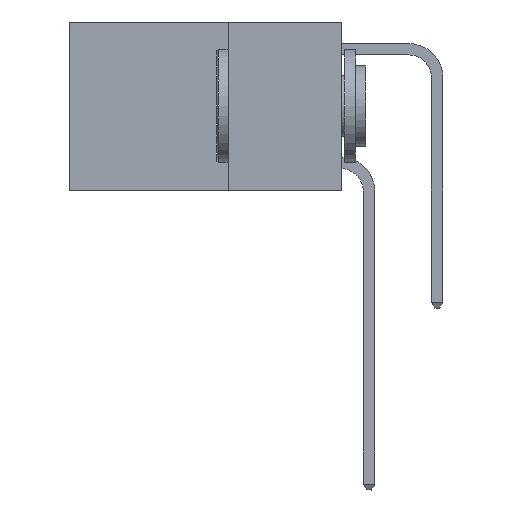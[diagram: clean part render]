
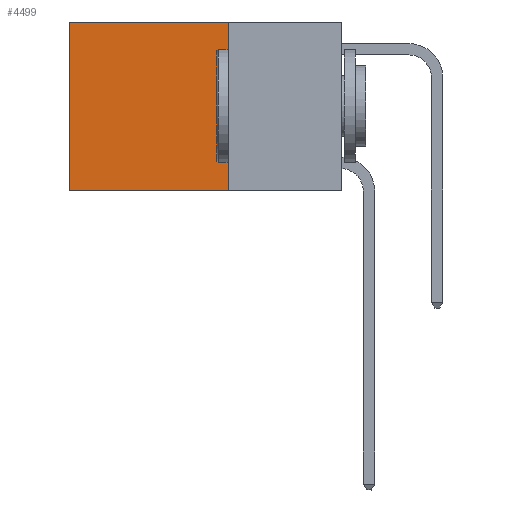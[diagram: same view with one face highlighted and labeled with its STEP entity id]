
A CAD part, left-side view. The second image highlights one B-rep face of the part: STEP entity #4499.
In plain terms, the highlighted planar face has unit normal (-1, 0, 0).
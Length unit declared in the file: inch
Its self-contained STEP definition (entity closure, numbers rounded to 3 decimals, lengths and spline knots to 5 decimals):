
#1267 = CARTESIAN_POINT ( 'NONE',  ( 0.2625, 0.25, -0.37 ) ) ;
#3978 = VECTOR ( 'NONE', #19620, 39.37008 ) ;
#4499 = ADVANCED_FACE ( 'NONE', ( #9199 ), #13347, .F. ) ;
#5817 = ORIENTED_EDGE ( 'NONE', *, *, #18738, .F. ) ;
#6195 = CARTESIAN_POINT ( 'NONE',  ( 0.2625, 0.25, 0. ) ) ;
#7428 = LINE ( 'NONE', #13682, #24692 ) ;
#7809 = CARTESIAN_POINT ( 'NONE',  ( 0.2625, 0.6, 0. ) ) ;
#7975 = LINE ( 'NONE', #7809, #18261 ) ;
#8742 = VERTEX_POINT ( 'NONE', #15320 ) ;
#9199 = FACE_OUTER_BOUND ( 'NONE', #31244, .T. ) ;
#9621 = CARTESIAN_POINT ( 'NONE',  ( 0.2625, 0.25, -0.37 ) ) ;
#10654 = EDGE_CURVE ( 'NONE', #8742, #15787, #7975, .T. ) ;
#12845 = ORIENTED_EDGE ( 'NONE', *, *, #21635, .F. ) ;
#13347 = PLANE ( 'NONE',  #19003 ) ;
#13682 = CARTESIAN_POINT ( 'NONE',  ( 0.2625, 0.25, 0. ) ) ;
#14117 = VECTOR ( 'NONE', #17431, 39.37008 ) ;
#15027 = CARTESIAN_POINT ( 'NONE',  ( 0.2625, 0.6, -0.37 ) ) ;
#15320 = CARTESIAN_POINT ( 'NONE',  ( 0.2625, 0.6, 0. ) ) ;
#15787 = VERTEX_POINT ( 'NONE', #15027 ) ;
#17431 = DIRECTION ( 'NONE',  ( 0., 1., 0. ) ) ;
#17470 = VERTEX_POINT ( 'NONE', #1267 ) ;
#17644 = ORIENTED_EDGE ( 'NONE', *, *, #26007, .T. ) ;
#18261 = VECTOR ( 'NONE', #31360, 39.37008 ) ;
#18738 = EDGE_CURVE ( 'NONE', #23819, #17470, #26959, .T. ) ;
#19003 = AXIS2_PLACEMENT_3D ( 'NONE', #32090, #26490, #21759 ) ;
#19620 = DIRECTION ( 'NONE',  ( 0., 0., -1. ) ) ;
#21116 = LINE ( 'NONE', #9621, #14117 ) ;
#21635 = EDGE_CURVE ( 'NONE', #17470, #15787, #21116, .T. ) ;
#21759 = DIRECTION ( 'NONE',  ( 0., 0., -1. ) ) ;
#23673 = CARTESIAN_POINT ( 'NONE',  ( 0.2625, 0.25, 0. ) ) ;
#23819 = VERTEX_POINT ( 'NONE', #23673 ) ;
#24692 = VECTOR ( 'NONE', #32080, 39.37008 ) ;
#26007 = EDGE_CURVE ( 'NONE', #23819, #8742, #7428, .T. ) ;
#26490 = DIRECTION ( 'NONE',  ( 1., 0., 0. ) ) ;
#26933 = ORIENTED_EDGE ( 'NONE', *, *, #10654, .T. ) ;
#26959 = LINE ( 'NONE', #6195, #3978 ) ;
#31244 = EDGE_LOOP ( 'NONE', ( #26933, #12845, #5817, #17644 ) ) ;
#31360 = DIRECTION ( 'NONE',  ( 0., 0., -1. ) ) ;
#32080 = DIRECTION ( 'NONE',  ( 0., 1., 0. ) ) ;
#32090 = CARTESIAN_POINT ( 'NONE',  ( 0.2625, 0.25, 0. ) ) ;
